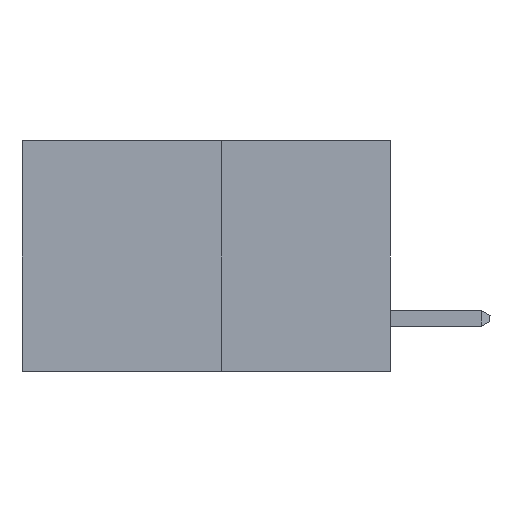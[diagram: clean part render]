
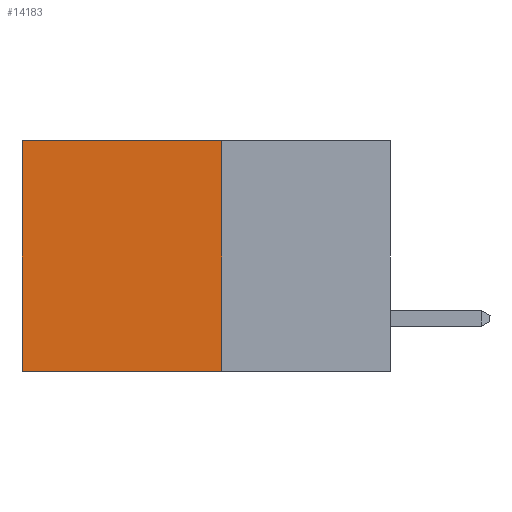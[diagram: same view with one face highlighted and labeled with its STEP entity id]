
A CAD part, left-side view. The second image highlights one B-rep face of the part: STEP entity #14183.
In plain terms, the highlighted planar face has unit normal (-1, 0, 0).
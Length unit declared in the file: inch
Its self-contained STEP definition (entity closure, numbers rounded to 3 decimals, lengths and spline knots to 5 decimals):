
#592 = DIRECTION ( 'NONE',  ( 0., 1., 0. ) ) ;
#974 = CARTESIAN_POINT ( 'NONE',  ( 0.277, 0.27, -0.37 ) ) ;
#1628 = EDGE_CURVE ( 'NONE', #4733, #5791, #17244, .T. ) ;
#1927 = EDGE_CURVE ( 'NONE', #10050, #13637, #12684, .T. ) ;
#4124 = LINE ( 'NONE', #4537, #4529 ) ;
#4128 = VECTOR ( 'NONE', #16016, 39.37008 ) ;
#4529 = VECTOR ( 'NONE', #14182, 39.37008 ) ;
#4537 = CARTESIAN_POINT ( 'NONE',  ( 0.277, 0.59, -0.37 ) ) ;
#4733 = VERTEX_POINT ( 'NONE', #5278 ) ;
#5278 = CARTESIAN_POINT ( 'NONE',  ( 0.277, 0.27, 0. ) ) ;
#5791 = VERTEX_POINT ( 'NONE', #9824 ) ;
#6595 = FACE_OUTER_BOUND ( 'NONE', #12171, .T. ) ;
#8061 = CARTESIAN_POINT ( 'NONE',  ( 0.277, 0.27, -0.37 ) ) ;
#8539 = VECTOR ( 'NONE', #592, 39.37008 ) ;
#8971 = ORIENTED_EDGE ( 'NONE', *, *, #11414, .F. ) ;
#9069 = EDGE_CURVE ( 'NONE', #5791, #13637, #4124, .T. ) ;
#9460 = PLANE ( 'NONE',  #12479 ) ;
#9824 = CARTESIAN_POINT ( 'NONE',  ( 0.277, 0.59, 0. ) ) ;
#10050 = VERTEX_POINT ( 'NONE', #14790 ) ;
#10055 = VECTOR ( 'NONE', #10388, 39.37008 ) ;
#10221 = CARTESIAN_POINT ( 'NONE',  ( 0.277, 0.27, 0. ) ) ;
#10388 = DIRECTION ( 'NONE',  ( 0., 1., 0. ) ) ;
#10848 = ORIENTED_EDGE ( 'NONE', *, *, #1628, .T. ) ;
#10874 = DIRECTION ( 'NONE',  ( 0., 0., -1. ) ) ;
#11414 = EDGE_CURVE ( 'NONE', #4733, #10050, #11866, .T. ) ;
#11866 = LINE ( 'NONE', #14723, #4128 ) ;
#12171 = EDGE_LOOP ( 'NONE', ( #16904, #17458, #8971, #10848 ) ) ;
#12479 = AXIS2_PLACEMENT_3D ( 'NONE', #8061, #14938, #10874 ) ;
#12684 = LINE ( 'NONE', #974, #8539 ) ;
#13603 = CARTESIAN_POINT ( 'NONE',  ( 0.277, 0.59, -0.37 ) ) ;
#13637 = VERTEX_POINT ( 'NONE', #13603 ) ;
#14182 = DIRECTION ( 'NONE',  ( 0., 0., -1. ) ) ;
#14183 = ADVANCED_FACE ( 'NONE', ( #6595 ), #9460, .F. ) ;
#14723 = CARTESIAN_POINT ( 'NONE',  ( 0.277, 0.27, -0.37 ) ) ;
#14790 = CARTESIAN_POINT ( 'NONE',  ( 0.277, 0.27, -0.37 ) ) ;
#14938 = DIRECTION ( 'NONE',  ( 1., 0., 0. ) ) ;
#16016 = DIRECTION ( 'NONE',  ( 0., 0., -1. ) ) ;
#16904 = ORIENTED_EDGE ( 'NONE', *, *, #9069, .T. ) ;
#17244 = LINE ( 'NONE', #10221, #10055 ) ;
#17458 = ORIENTED_EDGE ( 'NONE', *, *, #1927, .F. ) ;
